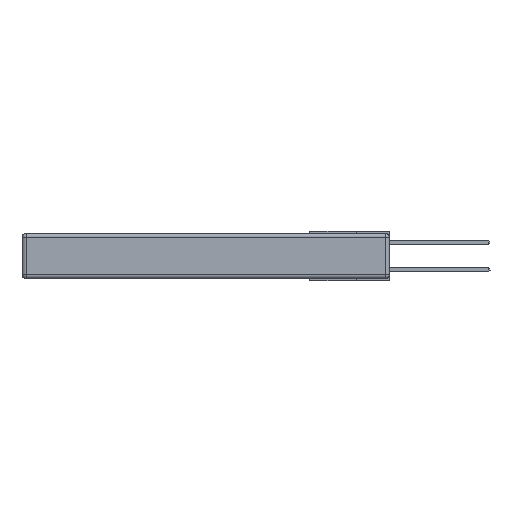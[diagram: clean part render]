
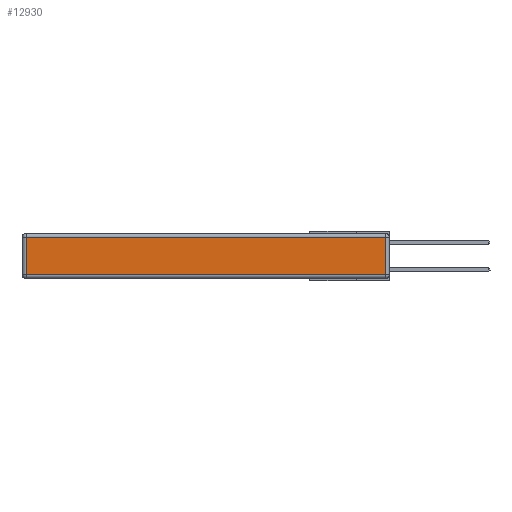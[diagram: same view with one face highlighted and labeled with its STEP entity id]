
A CAD part, left-side view. The second image highlights one B-rep face of the part: STEP entity #12930.
In plain terms, the highlighted planar face has unit normal (-1, 0, 0).
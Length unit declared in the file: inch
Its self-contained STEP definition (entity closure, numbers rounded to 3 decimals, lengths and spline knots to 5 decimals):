
#63 = CARTESIAN_POINT ( 'NONE',  ( 0., 2.75, -0.03 ) ) ;
#168 = LINE ( 'NONE', #2149, #16865 ) ;
#630 = EDGE_CURVE ( 'NONE', #16696, #1688, #16953, .T. ) ;
#831 = CARTESIAN_POINT ( 'NONE',  ( 0., 2.72, -0.343 ) ) ;
#1179 = DIRECTION ( 'NONE',  ( 0., 1., 0. ) ) ;
#1688 = VERTEX_POINT ( 'NONE', #13407 ) ;
#1760 = ORIENTED_EDGE ( 'NONE', *, *, #19754, .T. ) ;
#1784 = CARTESIAN_POINT ( 'NONE',  ( 0., 0., -0.313 ) ) ;
#2149 = CARTESIAN_POINT ( 'NONE',  ( 0., 0.03, -0.343 ) ) ;
#5200 = LINE ( 'NONE', #831, #5694 ) ;
#5499 = VECTOR ( 'NONE', #1179, 39.37008 ) ;
#5694 = VECTOR ( 'NONE', #15466, 39.37008 ) ;
#5937 = EDGE_CURVE ( 'NONE', #15278, #10246, #8163, .T. ) ;
#7140 = CARTESIAN_POINT ( 'NONE',  ( 0., 0., -0.343 ) ) ;
#8163 = LINE ( 'NONE', #1784, #19094 ) ;
#8172 = DIRECTION ( 'NONE',  ( 0., -1., 0. ) ) ;
#8492 = PLANE ( 'NONE',  #16235 ) ;
#10172 = CARTESIAN_POINT ( 'NONE',  ( 0., 0.03, -0.313 ) ) ;
#10246 = VERTEX_POINT ( 'NONE', #10172 ) ;
#10820 = EDGE_LOOP ( 'NONE', ( #14244, #1760, #19621, #13085 ) ) ;
#12175 = DIRECTION ( 'NONE',  ( -1., 0., 0. ) ) ;
#12930 = ADVANCED_FACE ( 'NONE', ( #17695 ), #8492, .T. ) ;
#13085 = ORIENTED_EDGE ( 'NONE', *, *, #14285, .T. ) ;
#13407 = CARTESIAN_POINT ( 'NONE',  ( 0., 2.72, -0.03 ) ) ;
#13795 = DIRECTION ( 'NONE',  ( 0., 0., 1. ) ) ;
#14244 = ORIENTED_EDGE ( 'NONE', *, *, #5937, .T. ) ;
#14285 = EDGE_CURVE ( 'NONE', #1688, #15278, #5200, .T. ) ;
#15278 = VERTEX_POINT ( 'NONE', #17010 ) ;
#15466 = DIRECTION ( 'NONE',  ( 0., 0., -1. ) ) ;
#16235 = AXIS2_PLACEMENT_3D ( 'NONE', #7140, #12175, #13795 ) ;
#16696 = VERTEX_POINT ( 'NONE', #18061 ) ;
#16865 = VECTOR ( 'NONE', #20069, 39.37008 ) ;
#16953 = LINE ( 'NONE', #63, #5499 ) ;
#17010 = CARTESIAN_POINT ( 'NONE',  ( 0., 2.72, -0.313 ) ) ;
#17695 = FACE_OUTER_BOUND ( 'NONE', #10820, .T. ) ;
#18061 = CARTESIAN_POINT ( 'NONE',  ( 0., 0.03, -0.03 ) ) ;
#19094 = VECTOR ( 'NONE', #8172, 39.37008 ) ;
#19621 = ORIENTED_EDGE ( 'NONE', *, *, #630, .T. ) ;
#19754 = EDGE_CURVE ( 'NONE', #10246, #16696, #168, .T. ) ;
#20069 = DIRECTION ( 'NONE',  ( 0., 0., 1. ) ) ;
